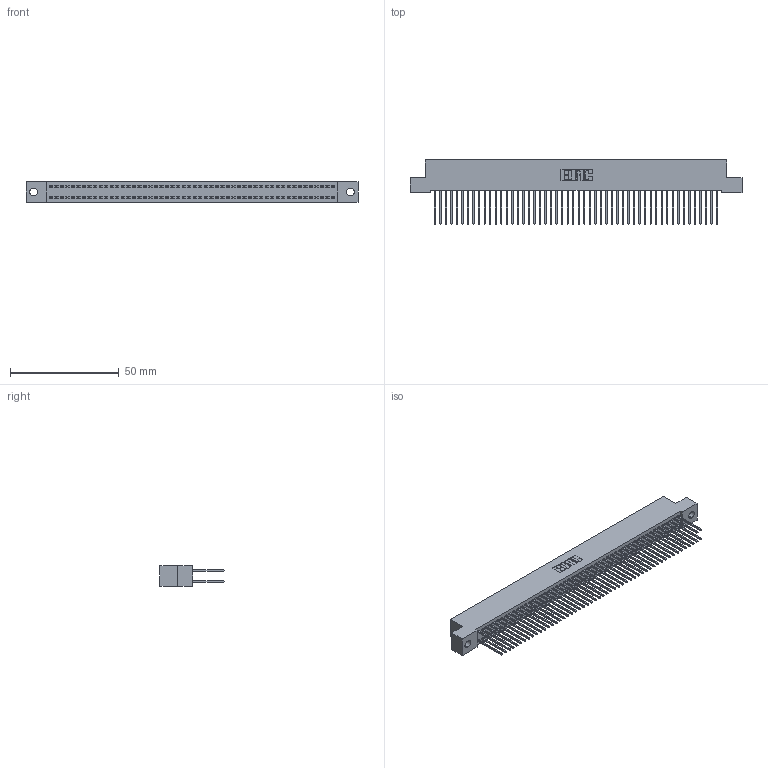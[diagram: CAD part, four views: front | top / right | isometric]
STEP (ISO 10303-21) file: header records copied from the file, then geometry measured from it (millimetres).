
FILE_DESCRIPTION (( 'STEP AP203' ), '1' );
FILE_NAME ('342-104-540-202.STEP', '2019-10-04T18:39:34', ( '' ), ( '' ), 'SwSTEP 2.0', 'SolidWorks 2016', '' );
FILE_SCHEMA (( 'CONFIG_CONTROL_DESIGN' ));
Length unit declared in the file: inch
Products named in the file (3): 342 Part_.128 Slot; 345-292-001_345-293-140; 342-104-540-202
Assembly tree (105 placements, depth 2):
  342-104-540-202
    342 Part_.128 Slot
    345-292-001_345-293-140  x104
Bounding box: 152.4 x 29.47 x 9.4 mm (x, y, z)
Volume: 14082.6 mm3; surface area: 24681.5 mm2
Topology: 105 solids, 105 shells, 5522 faces, 16431 edges, 10814 vertices
Faces by surface type: plane 3814, cylinder 1708
Entity records: 32181 total; most frequent: CARTESIAN_POINT 5322, ORIENTED_EDGE 5258, DIRECTION 4529, EDGE_CURVE 2629, VECTOR 2501, LINE 2501, VERTEX_POINT 1750, AXIS2_PLACEMENT_3D 1014
